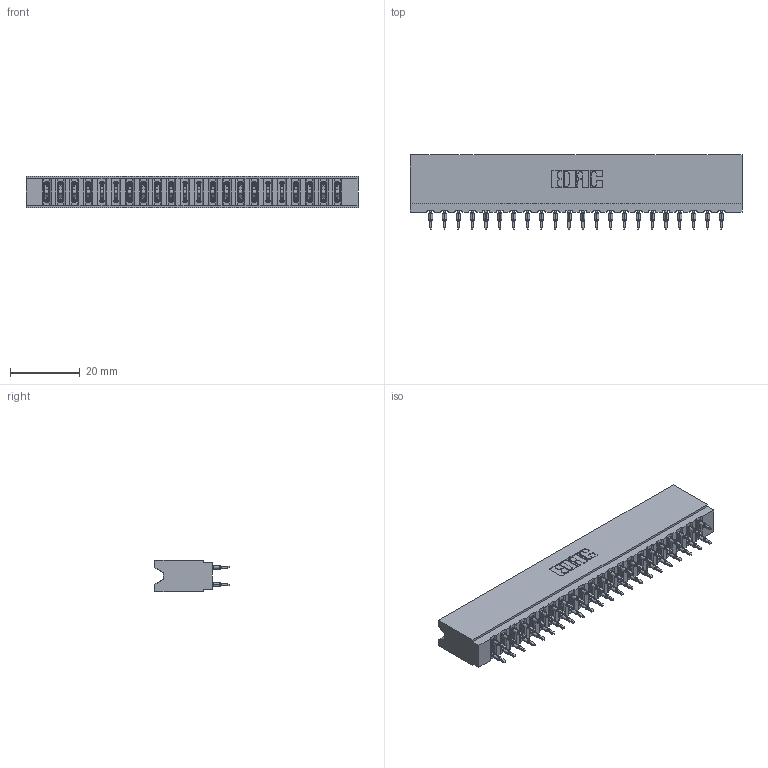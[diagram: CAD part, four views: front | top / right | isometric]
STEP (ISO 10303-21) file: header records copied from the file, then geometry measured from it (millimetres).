
FILE_DESCRIPTION (( 'STEP AP203' ), '1' );
FILE_NAME ('737-044-560-206.STEP', '2026-03-05T23:15:58', ( '' ), ( '' ), 'SwSTEP 2.0', 'SolidWorks 2023', '' );
FILE_SCHEMA (( 'CONFIG_CONTROL_DESIGN' ));
Length unit declared in the file: millimetre
Products named in the file (3): 737 Part_Insulator Option - 06; 745-292-001_560; 737-044-560-206
Assembly tree (45 placements, depth 2):
  737-044-560-206
    737 Part_Insulator Option - 06
    745-292-001_560  x44
Bounding box: 95.05 x 21.22 x 8.89 mm (x, y, z)
Volume: 9602.8 mm3; surface area: 14665.3 mm2
Topology: 45 solids, 45 shells, 4451 faces, 12181 edges, 7738 vertices
Faces by surface type: plane 2321, cylinder 986, bspline 880, torus 264
Entity records: 40804 total; most frequent: CARTESIAN_POINT 7594, ORIENTED_EDGE 6990, DIRECTION 6123, EDGE_CURVE 3495, LINE 3173, VECTOR 3173, VERTEX_POINT 2234, AXIS2_PLACEMENT_3D 1475
